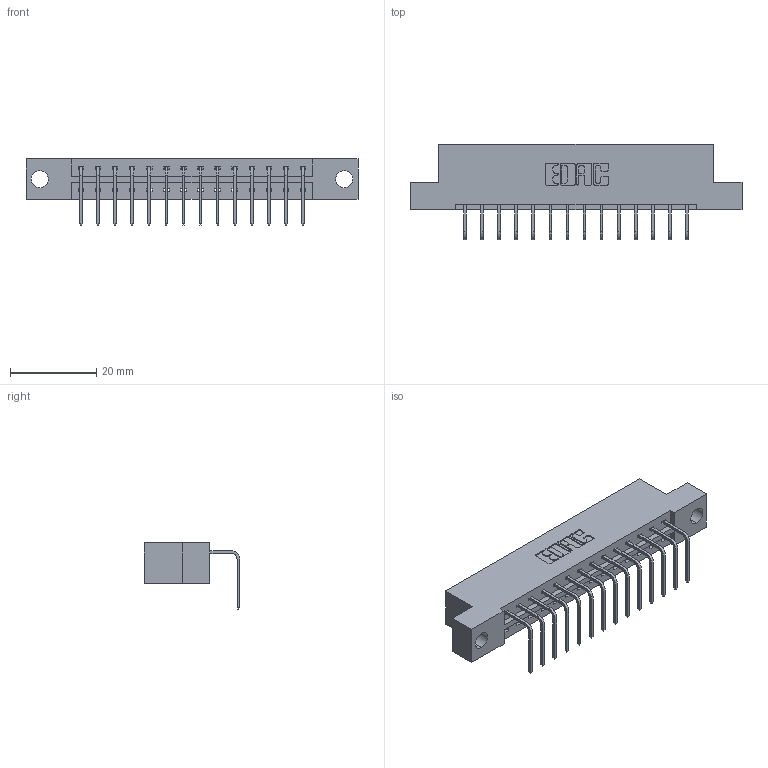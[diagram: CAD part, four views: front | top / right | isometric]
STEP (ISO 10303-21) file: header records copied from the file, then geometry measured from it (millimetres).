
FILE_DESCRIPTION (( 'STEP AP203' ), '1' );
FILE_NAME ('833-014-558-104.STEP', '2020-05-31T14:49:33', ( '' ), ( '' ), 'SwSTEP 2.0', 'SolidWorks 2020', '' );
FILE_SCHEMA (( 'CONFIG_CONTROL_DESIGN' ));
Length unit declared in the file: inch
Products named in the file (3): 833 Part_Flush - .156 Dia - TH; 345-292-001_558 Tail - 2; 833-014-558-104
Assembly tree (15 placements, depth 2):
  833-014-558-104
    833 Part_Flush - .156 Dia - TH
    345-292-001_558 Tail - 2  x14
Bounding box: 77.01 x 22.17 x 15.37 mm (x, y, z)
Volume: 7467.6 mm3; surface area: 7978 mm2
Topology: 15 solids, 15 shells, 954 faces, 2859 edges, 1886 vertices
Faces by surface type: plane 686, cylinder 268
Entity records: 12267 total; most frequent: CARTESIAN_POINT 2128, ORIENTED_EDGE 2078, DIRECTION 1851, EDGE_CURVE 1039, VECTOR 911, LINE 911, VERTEX_POINT 690, AXIS2_PLACEMENT_3D 470
